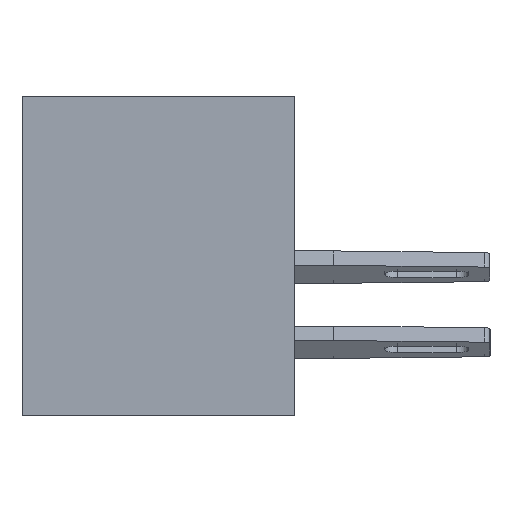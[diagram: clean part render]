
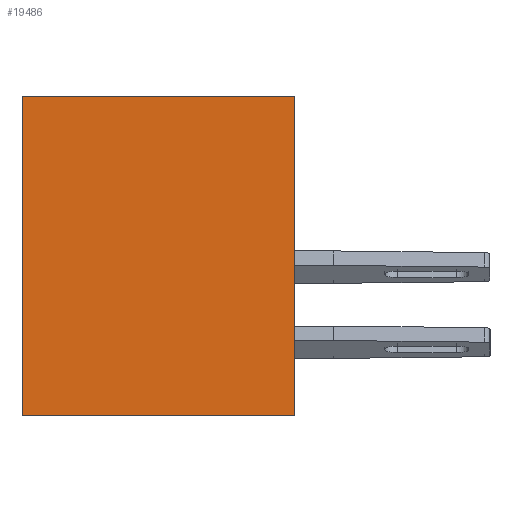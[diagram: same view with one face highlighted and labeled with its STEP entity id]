
A CAD part, left-side view. The second image highlights one B-rep face of the part: STEP entity #19486.
In plain terms, the highlighted planar face has unit normal (-1, 0, 0).
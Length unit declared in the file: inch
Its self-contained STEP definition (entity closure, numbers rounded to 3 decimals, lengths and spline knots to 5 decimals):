
#2237 = EDGE_CURVE ( 'NONE', #2317, #14116, #7222, .T. ) ;
#2317 = VERTEX_POINT ( 'NONE', #5472 ) ;
#2892 = FACE_OUTER_BOUND ( 'NONE', #5168, .T. ) ;
#2927 = ORIENTED_EDGE ( 'NONE', *, *, #17531, .T. ) ;
#3524 = AXIS2_PLACEMENT_3D ( 'NONE', #20887, #8045, #12221 ) ;
#5043 = VECTOR ( 'NONE', #12243, 39.37008 ) ;
#5168 = EDGE_LOOP ( 'NONE', ( #2927, #11080, #10646, #6554 ) ) ;
#5472 = CARTESIAN_POINT ( 'NONE',  ( 0., 0.453, 0. ) ) ;
#5549 = LINE ( 'NONE', #25999, #10521 ) ;
#5752 = CARTESIAN_POINT ( 'NONE',  ( 0., 0., 0. ) ) ;
#5757 = VERTEX_POINT ( 'NONE', #20078 ) ;
#5905 = EDGE_CURVE ( 'NONE', #5757, #8842, #9370, .T. ) ;
#6554 = ORIENTED_EDGE ( 'NONE', *, *, #5905, .T. ) ;
#7222 = LINE ( 'NONE', #22405, #26880 ) ;
#8045 = DIRECTION ( 'NONE',  ( 1., 0., 0. ) ) ;
#8423 = EDGE_CURVE ( 'NONE', #5757, #2317, #5549, .T. ) ;
#8842 = VERTEX_POINT ( 'NONE', #13463 ) ;
#9370 = LINE ( 'NONE', #25035, #5043 ) ;
#10521 = VECTOR ( 'NONE', #19498, 39.37008 ) ;
#10646 = ORIENTED_EDGE ( 'NONE', *, *, #8423, .F. ) ;
#11080 = ORIENTED_EDGE ( 'NONE', *, *, #2237, .F. ) ;
#12181 = CARTESIAN_POINT ( 'NONE',  ( 0., 0., 0. ) ) ;
#12221 = DIRECTION ( 'NONE',  ( 0., 0., -1. ) ) ;
#12243 = DIRECTION ( 'NONE',  ( 0., -1., 0. ) ) ;
#13463 = CARTESIAN_POINT ( 'NONE',  ( 0., 0., -0.531 ) ) ;
#14116 = VERTEX_POINT ( 'NONE', #5752 ) ;
#14322 = LINE ( 'NONE', #12181, #26986 ) ;
#14343 = DIRECTION ( 'NONE',  ( 0., 0., 1. ) ) ;
#17531 = EDGE_CURVE ( 'NONE', #8842, #14116, #14322, .T. ) ;
#19486 = ADVANCED_FACE ( 'NONE', ( #2892 ), #27218, .F. ) ;
#19498 = DIRECTION ( 'NONE',  ( 0., 0., 1. ) ) ;
#20078 = CARTESIAN_POINT ( 'NONE',  ( 0., 0.453, -0.531 ) ) ;
#20887 = CARTESIAN_POINT ( 'NONE',  ( 0., 0.453, 0. ) ) ;
#22405 = CARTESIAN_POINT ( 'NONE',  ( 0., 0.453, 0. ) ) ;
#25035 = CARTESIAN_POINT ( 'NONE',  ( 0., 0.453, -0.531 ) ) ;
#25999 = CARTESIAN_POINT ( 'NONE',  ( 0., 0.453, 0. ) ) ;
#26795 = DIRECTION ( 'NONE',  ( 0., -1., 0. ) ) ;
#26880 = VECTOR ( 'NONE', #26795, 39.37008 ) ;
#26986 = VECTOR ( 'NONE', #14343, 39.37008 ) ;
#27218 = PLANE ( 'NONE',  #3524 ) ;
